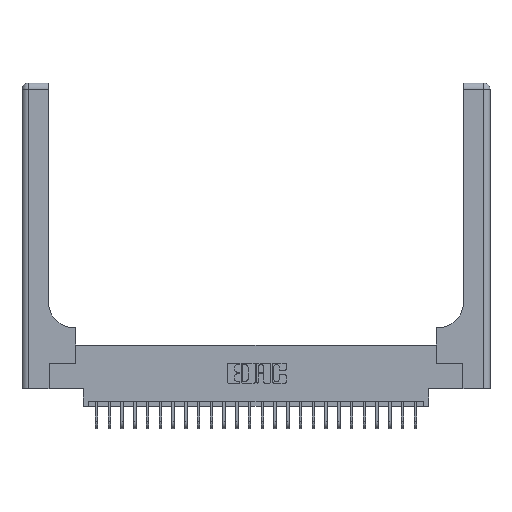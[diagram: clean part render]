
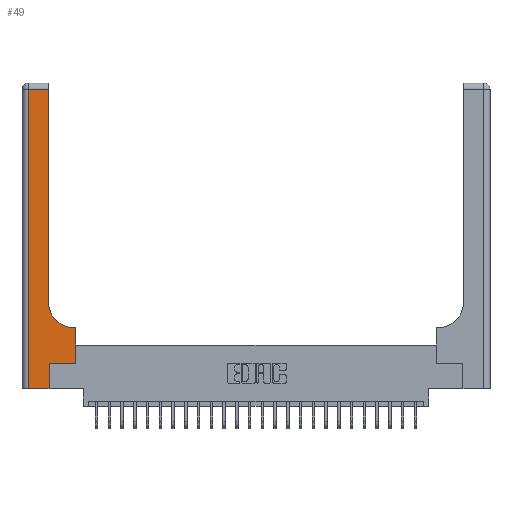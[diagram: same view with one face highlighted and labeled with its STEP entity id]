
A CAD part, top view. The second image highlights one B-rep face of the part: STEP entity #49.
In plain terms, the highlighted planar face has unit normal (0, 0, 1).
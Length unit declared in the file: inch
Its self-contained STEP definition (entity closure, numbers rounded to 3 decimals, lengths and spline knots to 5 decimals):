
#49 = ADVANCED_FACE ( 'NONE', ( #2819 ), #9156, .F. ) ;
#1088 = CARTESIAN_POINT ( 'NONE',  ( 0., 2.94, 0.37 ) ) ;
#1216 = DIRECTION ( 'NONE',  ( -1., 0., 0. ) ) ;
#1975 = LINE ( 'NONE', #14149, #9709 ) ;
#2323 = VERTEX_POINT ( 'NONE', #9271 ) ;
#2819 = FACE_OUTER_BOUND ( 'NONE', #7186, .T. ) ;
#2953 = CARTESIAN_POINT ( 'NONE',  ( 0., 3., 0.37 ) ) ;
#3596 = EDGE_CURVE ( 'NONE', #21424, #2323, #17950, .T. ) ;
#3689 = VECTOR ( 'NONE', #9413, 39.37008 ) ;
#3724 = EDGE_CURVE ( 'NONE', #21317, #21424, #1975, .T. ) ;
#3908 = AXIS2_PLACEMENT_3D ( 'NONE', #2953, #7010, #6759 ) ;
#4082 = DIRECTION ( 'NONE',  ( 0., 0., -1. ) ) ;
#4296 = EDGE_CURVE ( 'NONE', #9127, #21317, #23157, .T. ) ;
#4456 = LINE ( 'NONE', #20549, #17887 ) ;
#4766 = CARTESIAN_POINT ( 'NONE',  ( 0.06, 2.94, 0.37 ) ) ;
#5138 = CARTESIAN_POINT ( 'NONE',  ( 0.265, 0., 0.37 ) ) ;
#5802 = CARTESIAN_POINT ( 'NONE',  ( 0.06, 0., 0.37 ) ) ;
#6759 = DIRECTION ( 'NONE',  ( -1., 0., 0. ) ) ;
#7010 = DIRECTION ( 'NONE',  ( 0., 0., -1. ) ) ;
#7173 = LINE ( 'NONE', #1088, #14807 ) ;
#7186 = EDGE_LOOP ( 'NONE', ( #22322, #10310, #23602, #15694, #10059, #24927, #26264, #15908, #20779 ) ) ;
#7781 = DIRECTION ( 'NONE',  ( 1., 0., 0. ) ) ;
#8496 = VERTEX_POINT ( 'NONE', #4766 ) ;
#8556 = CARTESIAN_POINT ( 'NONE',  ( 0.528, 0.25, 0.37 ) ) ;
#9127 = VERTEX_POINT ( 'NONE', #5138 ) ;
#9156 = PLANE ( 'NONE',  #3908 ) ;
#9271 = CARTESIAN_POINT ( 'NONE',  ( 0.528, 0.6, 0.37 ) ) ;
#9413 = DIRECTION ( 'NONE',  ( -1., 0., 0. ) ) ;
#9709 = VECTOR ( 'NONE', #7781, 39.37008 ) ;
#9775 = DIRECTION ( 'NONE',  ( 1., 0., 0. ) ) ;
#10059 = ORIENTED_EDGE ( 'NONE', *, *, #4296, .T. ) ;
#10087 = CARTESIAN_POINT ( 'NONE',  ( 0., 0., 0.37 ) ) ;
#10310 = ORIENTED_EDGE ( 'NONE', *, *, #19773, .T. ) ;
#10406 = CARTESIAN_POINT ( 'NONE',  ( 0.26, 2.94, 0.37 ) ) ;
#12263 = VECTOR ( 'NONE', #15808, 39.37008 ) ;
#12836 = EDGE_CURVE ( 'NONE', #8496, #14069, #18231, .T. ) ;
#13418 = VERTEX_POINT ( 'NONE', #14817 ) ;
#14069 = VERTEX_POINT ( 'NONE', #5802 ) ;
#14149 = CARTESIAN_POINT ( 'NONE',  ( 0.265, 0.25, 0.37 ) ) ;
#14210 = VECTOR ( 'NONE', #25163, 39.37008 ) ;
#14413 = EDGE_CURVE ( 'NONE', #14069, #9127, #24005, .T. ) ;
#14807 = VECTOR ( 'NONE', #1216, 39.37008 ) ;
#14817 = CARTESIAN_POINT ( 'NONE',  ( 0.51, 0.6, 0.37 ) ) ;
#15694 = ORIENTED_EDGE ( 'NONE', *, *, #14413, .T. ) ;
#15808 = DIRECTION ( 'NONE',  ( 0., -1., 0. ) ) ;
#15908 = ORIENTED_EDGE ( 'NONE', *, *, #22599, .T. ) ;
#16042 = DIRECTION ( 'NONE',  ( 1., 0., 0. ) ) ;
#16171 = VECTOR ( 'NONE', #19560, 39.37008 ) ;
#16407 = CARTESIAN_POINT ( 'NONE',  ( 0.265, 0.25, 0.37 ) ) ;
#16803 = CARTESIAN_POINT ( 'NONE',  ( 0.265, 0., 0.37 ) ) ;
#17129 = VERTEX_POINT ( 'NONE', #10406 ) ;
#17683 = CARTESIAN_POINT ( 'NONE',  ( 0.26, 0.6, 0.37 ) ) ;
#17887 = VECTOR ( 'NONE', #22700, 39.37008 ) ;
#17950 = LINE ( 'NONE', #21989, #16171 ) ;
#18231 = LINE ( 'NONE', #26179, #12263 ) ;
#18290 = CARTESIAN_POINT ( 'NONE',  ( 0.51, 0.85, 0.37 ) ) ;
#18338 = VECTOR ( 'NONE', #16042, 39.37008 ) ;
#19292 = AXIS2_PLACEMENT_3D ( 'NONE', #18290, #4082, #9775 ) ;
#19560 = DIRECTION ( 'NONE',  ( 0., 1., 0. ) ) ;
#19773 = EDGE_CURVE ( 'NONE', #17129, #8496, #7173, .T. ) ;
#20196 = CIRCLE ( 'NONE', #19292, 0.25 ) ;
#20504 = EDGE_CURVE ( 'NONE', #24829, #17129, #4456, .T. ) ;
#20549 = CARTESIAN_POINT ( 'NONE',  ( 0.26, 3., 0.37 ) ) ;
#20779 = ORIENTED_EDGE ( 'NONE', *, *, #25863, .T. ) ;
#21317 = VERTEX_POINT ( 'NONE', #16407 ) ;
#21424 = VERTEX_POINT ( 'NONE', #8556 ) ;
#21989 = CARTESIAN_POINT ( 'NONE',  ( 0.528, 0.25, 0.37 ) ) ;
#22322 = ORIENTED_EDGE ( 'NONE', *, *, #20504, .T. ) ;
#22599 = EDGE_CURVE ( 'NONE', #2323, #13418, #24256, .T. ) ;
#22700 = DIRECTION ( 'NONE',  ( 0., 1., 0. ) ) ;
#23157 = LINE ( 'NONE', #16803, #14210 ) ;
#23602 = ORIENTED_EDGE ( 'NONE', *, *, #12836, .T. ) ;
#24005 = LINE ( 'NONE', #10087, #18338 ) ;
#24256 = LINE ( 'NONE', #17683, #3689 ) ;
#24829 = VERTEX_POINT ( 'NONE', #25521 ) ;
#24927 = ORIENTED_EDGE ( 'NONE', *, *, #3724, .T. ) ;
#25163 = DIRECTION ( 'NONE',  ( 0., 1., 0. ) ) ;
#25521 = CARTESIAN_POINT ( 'NONE',  ( 0.26, 0.85, 0.37 ) ) ;
#25863 = EDGE_CURVE ( 'NONE', #13418, #24829, #20196, .T. ) ;
#26179 = CARTESIAN_POINT ( 'NONE',  ( 0.06, 3., 0.37 ) ) ;
#26264 = ORIENTED_EDGE ( 'NONE', *, *, #3596, .T. ) ;
